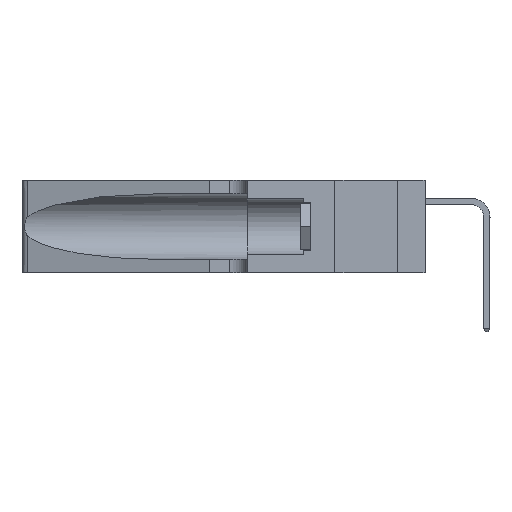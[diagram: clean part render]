
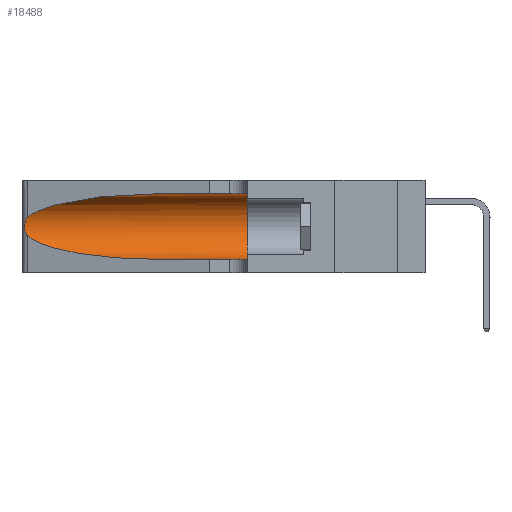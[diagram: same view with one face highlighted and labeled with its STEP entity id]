
A CAD part, left-side view. The second image highlights one B-rep face of the part: STEP entity #18488.
In plain terms, the highlighted cylindrical face has radius 3.308 mm (diameter 6.617 mm), a partial arc.
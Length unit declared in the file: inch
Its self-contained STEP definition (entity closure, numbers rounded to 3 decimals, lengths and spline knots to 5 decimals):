
#97 = CARTESIAN_POINT ( 'NONE',  ( 0.25555, 1.22994, 0.2215 ) ) ;
#492 = ORIENTED_EDGE ( 'NONE', *, *, #32079, .T. ) ;
#1707 = ORIENTED_EDGE ( 'NONE', *, *, #23658, .T. ) ;
#2264 = DIRECTION ( 'NONE',  ( 0., -1., 0. ) ) ;
#2689 = CARTESIAN_POINT ( 'NONE',  ( 0.25487, 1.22718, 0.14631 ) ) ;
#3158 =( BOUNDED_CURVE ( )  B_SPLINE_CURVE ( 3, ( #2689, #21169, #11986, #33401 ),
 .UNSPECIFIED., .F., .T. ) 
 B_SPLINE_CURVE_WITH_KNOTS ( ( 4, 4 ),
 ( 3.44316, 4.71239 ),
 .UNSPECIFIED. ) 
 CURVE ( )  GEOMETRIC_REPRESENTATION_ITEM ( )  RATIONAL_B_SPLINE_CURVE ( ( 1., 0.87, 0.87, 1. ) ) 
 REPRESENTATION_ITEM ( '' )  );
#3188 = CARTESIAN_POINT ( 'NONE',  ( 0.25787, 1.23484, 0.2124 ) ) ;
#3562 = CARTESIAN_POINT ( 'NONE',  ( 0.1305, 1.61858, 0.185 ) ) ;
#3719 = VERTEX_POINT ( 'NONE', #32669 ) ;
#6287 = CARTESIAN_POINT ( 'NONE',  ( 0.26018, 1.23835, 0.19895 ) ) ;
#6575 = ORIENTED_EDGE ( 'NONE', *, *, #34414, .T. ) ;
#6653 = CIRCLE ( 'NONE', #15417, 0.13025 ) ;
#6662 = DIRECTION ( 'NONE',  ( 0., 0., -1. ) ) ;
#9391 = CARTESIAN_POINT ( 'NONE',  ( 0.25487, 1.22718, 0.22369 ) ) ;
#9396 = CARTESIAN_POINT ( 'NONE',  ( 0.26075, 1.23896, 0.178 ) ) ;
#9504 = VECTOR ( 'NONE', #16133, 39.37008 ) ;
#9561 = EDGE_CURVE ( 'NONE', #3719, #32394, #6653, .T. ) ;
#10346 =( BOUNDED_CURVE ( )  B_SPLINE_CURVE ( 3, ( #18577, #36742, #27760, #9391 ),
 .UNSPECIFIED., .F., .T. ) 
 B_SPLINE_CURVE_WITH_KNOTS ( ( 4, 4 ),
 ( 1.5708, 2.84003 ),
 .UNSPECIFIED. ) 
 CURVE ( )  GEOMETRIC_REPRESENTATION_ITEM ( )  RATIONAL_B_SPLINE_CURVE ( ( 1., 0.87, 0.87, 1. ) ) 
 REPRESENTATION_ITEM ( '' )  );
#11123 = EDGE_CURVE ( 'NONE', #36295, #15875, #31685, .T. ) ;
#11373 = CARTESIAN_POINT ( 'NONE',  ( 0.25487, 1.22718, 0.14631 ) ) ;
#11518 = DIRECTION ( 'NONE',  ( 0., 1., 0. ) ) ;
#11986 = CARTESIAN_POINT ( 'NONE',  ( 0.18966, 0.96281, 0.05475 ) ) ;
#12476 = CARTESIAN_POINT ( 'NONE',  ( 0.25856, 1.23593, 0.16098 ) ) ;
#13620 = ORIENTED_EDGE ( 'NONE', *, *, #11123, .T. ) ;
#14443 = CARTESIAN_POINT ( 'NONE',  ( 0.25487, 1.22718, 0.22369 ) ) ;
#15417 = AXIS2_PLACEMENT_3D ( 'NONE', #29878, #11518, #32939 ) ;
#15598 = CARTESIAN_POINT ( 'NONE',  ( 0.25639, 1.23186, 0.15144 ) ) ;
#15875 = VERTEX_POINT ( 'NONE', #11373 ) ;
#16133 = DIRECTION ( 'NONE',  ( 0., -1., 0. ) ) ;
#16429 = CARTESIAN_POINT ( 'NONE',  ( 0.1305, 0.35, 0.05475 ) ) ;
#17852 = LINE ( 'NONE', #38879, #25992 ) ;
#18488 = ADVANCED_FACE ( 'NONE', ( #24191 ), #23248, .F. ) ;
#18577 = CARTESIAN_POINT ( 'NONE',  ( 0.1305, 0.72297, 0.31525 ) ) ;
#18710 = CARTESIAN_POINT ( 'NONE',  ( 0.25487, 1.22718, 0.14631 ) ) ;
#21169 = CARTESIAN_POINT ( 'NONE',  ( 0.2373, 1.15595, 0.08982 ) ) ;
#21644 = CARTESIAN_POINT ( 'NONE',  ( 0.25487, 1.22718, 0.22369 ) ) ;
#23248 = CYLINDRICAL_SURFACE ( 'NONE', #35061, 0.13025 ) ;
#23658 = EDGE_CURVE ( 'NONE', #36412, #32394, #17852, .T. ) ;
#23731 = EDGE_LOOP ( 'NONE', ( #6575, #13620, #492, #1707, #26034, #35206 ) ) ;
#23806 = VERTEX_POINT ( 'NONE', #24590 ) ;
#24191 = FACE_OUTER_BOUND ( 'NONE', #23731, .T. ) ;
#24590 = CARTESIAN_POINT ( 'NONE',  ( 0.1305, 0.72297, 0.31525 ) ) ;
#24723 = CARTESIAN_POINT ( 'NONE',  ( 0.25854, 1.2359, 0.20912 ) ) ;
#25108 = DIRECTION ( 'NONE',  ( 0., -1., 0. ) ) ;
#25992 = VECTOR ( 'NONE', #2264, 39.37008 ) ;
#26034 = ORIENTED_EDGE ( 'NONE', *, *, #9561, .F. ) ;
#27760 = CARTESIAN_POINT ( 'NONE',  ( 0.2373, 1.15595, 0.28018 ) ) ;
#27762 = CARTESIAN_POINT ( 'NONE',  ( 0.26075, 1.23896, 0.19203 ) ) ;
#29074 = EDGE_CURVE ( 'NONE', #23806, #3719, #33913, .T. ) ;
#29878 = CARTESIAN_POINT ( 'NONE',  ( 0.1305, 0.35, 0.185 ) ) ;
#30355 = CARTESIAN_POINT ( 'NONE',  ( 0.1305, 0.72297, 0.05475 ) ) ;
#30830 = CARTESIAN_POINT ( 'NONE',  ( 0.26017, 1.23833, 0.17102 ) ) ;
#31685 = B_SPLINE_CURVE_WITH_KNOTS ( 'NONE', 3,
 ( #21644, #97, #36746, #3188, #24723, #6287, #27762, #9396, #30830, #12476, #33869, #15598, #36874, #18710 ),
 .UNSPECIFIED., .F., .F.,
 ( 4, 2, 2, 2, 2, 2, 4 ),
 ( 0., 0.00027, 0.00053, 0.00107, 0.0016, 0.00187, 0.00214 ),
 .UNSPECIFIED. ) ;
#32079 = EDGE_CURVE ( 'NONE', #15875, #36412, #3158, .T. ) ;
#32394 = VERTEX_POINT ( 'NONE', #16429 ) ;
#32669 = CARTESIAN_POINT ( 'NONE',  ( 0.1305, 0.35, 0.31525 ) ) ;
#32939 = DIRECTION ( 'NONE',  ( 0., 0., 1. ) ) ;
#33401 = CARTESIAN_POINT ( 'NONE',  ( 0.1305, 0.72297, 0.05475 ) ) ;
#33869 = CARTESIAN_POINT ( 'NONE',  ( 0.25789, 1.23486, 0.15765 ) ) ;
#33913 = LINE ( 'NONE', #34401, #9504 ) ;
#34401 = CARTESIAN_POINT ( 'NONE',  ( 0.1305, 1.61858, 0.31525 ) ) ;
#34414 = EDGE_CURVE ( 'NONE', #23806, #36295, #10346, .T. ) ;
#35061 = AXIS2_PLACEMENT_3D ( 'NONE', #3562, #25108, #6662 ) ;
#35206 = ORIENTED_EDGE ( 'NONE', *, *, #29074, .F. ) ;
#36295 = VERTEX_POINT ( 'NONE', #14443 ) ;
#36412 = VERTEX_POINT ( 'NONE', #30355 ) ;
#36742 = CARTESIAN_POINT ( 'NONE',  ( 0.18966, 0.96281, 0.31525 ) ) ;
#36746 = CARTESIAN_POINT ( 'NONE',  ( 0.25639, 1.23184, 0.21858 ) ) ;
#36874 = CARTESIAN_POINT ( 'NONE',  ( 0.25555, 1.22993, 0.14849 ) ) ;
#38879 = CARTESIAN_POINT ( 'NONE',  ( 0.1305, 1.61858, 0.05475 ) ) ;
